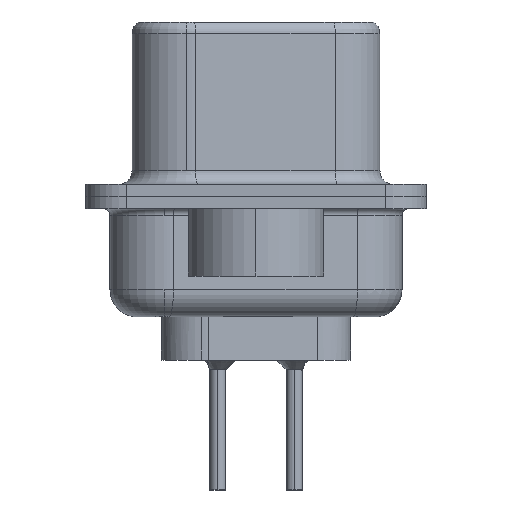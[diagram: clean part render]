
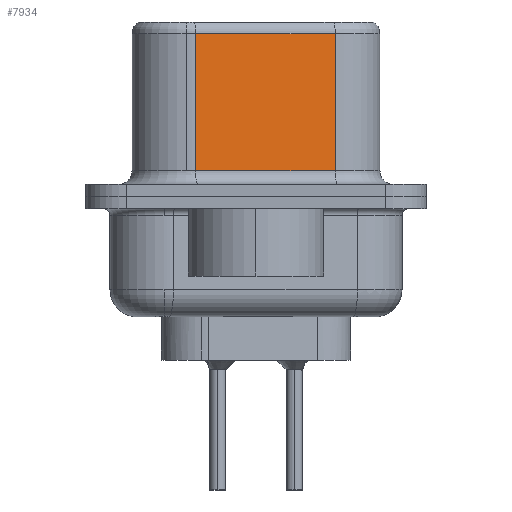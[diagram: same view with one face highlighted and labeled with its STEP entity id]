
A CAD part, left-side view. The second image highlights one B-rep face of the part: STEP entity #7934.
In plain terms, the highlighted planar face has unit normal (-0.985, -0.174, 0).
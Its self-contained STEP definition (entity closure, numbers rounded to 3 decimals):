
#629 = LINE ( 'NONE', #7198, #9709 ) ;
#1779 = DIRECTION ( 'NONE',  ( 0.174, -0.985, 0. ) ) ;
#2413 = ORIENTED_EDGE ( 'NONE', *, *, #10045, .T. ) ;
#2973 = DIRECTION ( 'NONE',  ( 0.985, 0.174, 0. ) ) ;
#3322 = LINE ( 'NONE', #8516, #16279 ) ;
#4033 = CARTESIAN_POINT ( 'NONE',  ( 4.575, -2.927, 6.02 ) ) ;
#5323 = LINE ( 'NONE', #8794, #5712 ) ;
#5692 = DIRECTION ( 'NONE',  ( 0., 0., -1. ) ) ;
#5712 = VECTOR ( 'NONE', #1779, 1000. ) ;
#6899 = VERTEX_POINT ( 'NONE', #12136 ) ;
#7198 = CARTESIAN_POINT ( 'NONE',  ( 4.575, -2.927, 6.02 ) ) ;
#7711 = CARTESIAN_POINT ( 'NONE',  ( 3.665, 2.233, 0.95 ) ) ;
#7934 = ADVANCED_FACE ( 'NONE', ( #19051 ), #15817, .F. ) ;
#8295 = DIRECTION ( 'NONE',  ( 0., 0., -1. ) ) ;
#8516 = CARTESIAN_POINT ( 'NONE',  ( 3.665, 2.233, 6.52 ) ) ;
#8794 = CARTESIAN_POINT ( 'NONE',  ( 4.575, -2.927, 0.95 ) ) ;
#8809 = EDGE_CURVE ( 'NONE', #19477, #6899, #629, .T. ) ;
#8828 = ORIENTED_EDGE ( 'NONE', *, *, #17867, .T. ) ;
#9264 = CARTESIAN_POINT ( 'NONE',  ( 4.575, -2.927, 6.52 ) ) ;
#9363 = DIRECTION ( 'NONE',  ( -0.174, 0.985, 0. ) ) ;
#9709 = VECTOR ( 'NONE', #13786, 1000. ) ;
#10045 = EDGE_CURVE ( 'NONE', #6899, #19023, #3322, .T. ) ;
#10701 = CARTESIAN_POINT ( 'NONE',  ( 4.575, -2.927, 0.95 ) ) ;
#10993 = AXIS2_PLACEMENT_3D ( 'NONE', #21196, #2973, #9363 ) ;
#12136 = CARTESIAN_POINT ( 'NONE',  ( 3.665, 2.233, 6.02 ) ) ;
#12270 = ORIENTED_EDGE ( 'NONE', *, *, #14446, .F. ) ;
#13786 = DIRECTION ( 'NONE',  ( -0.174, 0.985, 0. ) ) ;
#13923 = VERTEX_POINT ( 'NONE', #10701 ) ;
#14269 = EDGE_LOOP ( 'NONE', ( #12270, #14493, #2413, #8828 ) ) ;
#14446 = EDGE_CURVE ( 'NONE', #19477, #13923, #15608, .T. ) ;
#14493 = ORIENTED_EDGE ( 'NONE', *, *, #8809, .T. ) ;
#15608 = LINE ( 'NONE', #9264, #17000 ) ;
#15817 = PLANE ( 'NONE',  #10993 ) ;
#16279 = VECTOR ( 'NONE', #8295, 1000. ) ;
#17000 = VECTOR ( 'NONE', #5692, 1000. ) ;
#17867 = EDGE_CURVE ( 'NONE', #19023, #13923, #5323, .T. ) ;
#19023 = VERTEX_POINT ( 'NONE', #7711 ) ;
#19051 = FACE_OUTER_BOUND ( 'NONE', #14269, .T. ) ;
#19477 = VERTEX_POINT ( 'NONE', #4033 ) ;
#21196 = CARTESIAN_POINT ( 'NONE',  ( 4.575, -2.927, 6.52 ) ) ;
